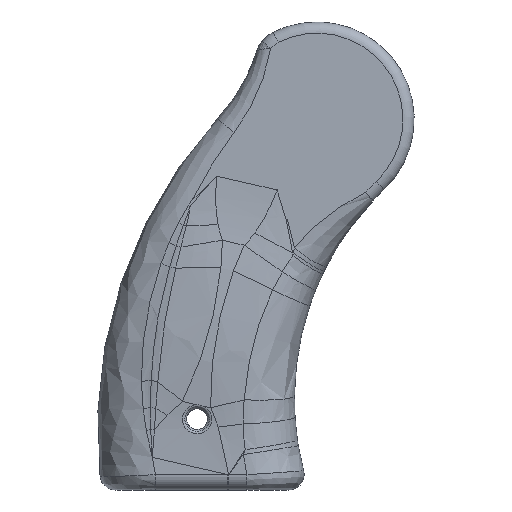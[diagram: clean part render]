
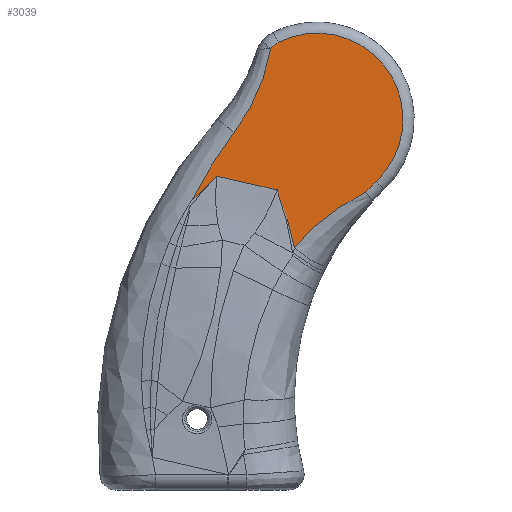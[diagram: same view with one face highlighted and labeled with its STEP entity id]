
A CAD part, front view. The second image highlights one B-rep face of the part: STEP entity #3039.
In plain terms, the highlighted planar face has unit normal (0, -1, 0).
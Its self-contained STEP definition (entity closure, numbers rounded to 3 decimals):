
#44=PLANE('',#3311);
#94=LINE('',#7707,#159);
#159=VECTOR('',#3801,10.);
#391=FACE_OUTER_BOUND('',#596,.T.);
#596=EDGE_LOOP('',(#2547,#2548,#2549,#2550,#2551,#2552,#2553,#2554,#2555,
#2556));
#791=B_SPLINE_CURVE_WITH_KNOTS('',3,(#7424,#7425,#7426,#7427,#7428,#7429),
 .UNSPECIFIED.,.F.,.F.,(4,2,4),(-1.76,-1.755,-0.68),
 .UNSPECIFIED.);
#835=B_SPLINE_CURVE_WITH_KNOTS('',3,(#8230,#8231,#8232,#8233,#8234),
 .UNSPECIFIED.,.F.,.F.,(4,1,4),(0.198,0.358,0.476),
 .UNSPECIFIED.);
#838=B_SPLINE_CURVE_WITH_KNOTS('',3,(#8290,#8291,#8292,#8293,#8294,#8295),
 .UNSPECIFIED.,.F.,.F.,(4,2,4),(-0.338,0.,1.319),
 .UNSPECIFIED.);
#848=B_SPLINE_CURVE_WITH_KNOTS('',3,(#8391,#8392,#8393,#8394),
 .UNSPECIFIED.,.F.,.F.,(4,4),(1.319,2.734),
 .UNSPECIFIED.);
#850=B_SPLINE_CURVE_WITH_KNOTS('',3,(#8456,#8457,#8458,#8459,#8460,#8461),
 .UNSPECIFIED.,.F.,.F.,(4,2,4),(0.142,0.227,0.228),
 .UNSPECIFIED.);
#851=B_SPLINE_CURVE_WITH_KNOTS('',3,(#8462,#8463,#8464,#8465,#8466,#8467),
 .UNSPECIFIED.,.F.,.F.,(4,2,4),(-0.507,0.,0.005),
 .UNSPECIFIED.);
#1024=CIRCLE('',#3304,15.352);
#1026=CIRCLE('',#3307,53.538);
#1028=CIRCLE('',#3310,4.);
#1262=VERTEX_POINT('',#7418);
#1263=VERTEX_POINT('',#7423);
#1282=VERTEX_POINT('',#7706);
#1298=VERTEX_POINT('',#8108);
#1299=VERTEX_POINT('',#8110);
#1300=VERTEX_POINT('',#8114);
#1301=VERTEX_POINT('',#8271);
#1302=VERTEX_POINT('',#8282);
#1311=VERTEX_POINT('',#8386);
#1312=VERTEX_POINT('',#8455);
#1665=EDGE_CURVE('',#1263,#1262,#791,.T.);
#1693=EDGE_CURVE('',#1282,#1263,#94,.T.);
#1721=EDGE_CURVE('',#1299,#1298,#1024,.T.);
#1724=EDGE_CURVE('',#1300,#1299,#1026,.T.);
#1725=EDGE_CURVE('',#1262,#1300,#835,.T.);
#1728=EDGE_CURVE('',#1301,#1302,#838,.T.);
#1738=EDGE_CURVE('',#1302,#1311,#848,.T.);
#1741=EDGE_CURVE('',#1298,#1301,#1028,.T.);
#1742=EDGE_CURVE('',#1312,#1311,#850,.T.);
#1743=EDGE_CURVE('',#1312,#1282,#851,.T.);
#2547=ORIENTED_EDGE('',*,*,#1742,.F.);
#2548=ORIENTED_EDGE('',*,*,#1743,.T.);
#2549=ORIENTED_EDGE('',*,*,#1693,.T.);
#2550=ORIENTED_EDGE('',*,*,#1665,.T.);
#2551=ORIENTED_EDGE('',*,*,#1725,.T.);
#2552=ORIENTED_EDGE('',*,*,#1724,.T.);
#2553=ORIENTED_EDGE('',*,*,#1721,.T.);
#2554=ORIENTED_EDGE('',*,*,#1741,.T.);
#2555=ORIENTED_EDGE('',*,*,#1728,.T.);
#2556=ORIENTED_EDGE('',*,*,#1738,.T.);
#3039=ADVANCED_FACE('',(#391),#44,.F.);
#3304=AXIS2_PLACEMENT_3D('',#8111,#3814,#3815);
#3307=AXIS2_PLACEMENT_3D('',#8194,#3820,#3821);
#3310=AXIS2_PLACEMENT_3D('',#8453,#3826,#3827);
#3311=AXIS2_PLACEMENT_3D('',#8454,#3828,#3829);
#3801=DIRECTION('',(0.975,0.,-0.222));
#3814=DIRECTION('center_axis',(0.,-1.,0.));
#3815=DIRECTION('ref_axis',(0.78,0.,0.626));
#3820=DIRECTION('center_axis',(0.,1.,0.));
#3821=DIRECTION('ref_axis',(0.69,0.,-0.724));
#3826=DIRECTION('center_axis',(0.,-1.,0.));
#3827=DIRECTION('ref_axis',(-0.63,0.,0.777));
#3828=DIRECTION('center_axis',(0.,1.,0.));
#3829=DIRECTION('ref_axis',(1.,0.,0.));
#7418=CARTESIAN_POINT('',(17.65,-6.75,40.273));
#7423=CARTESIAN_POINT('',(14.585,-6.75,50.63));
#7424=CARTESIAN_POINT('Ctrl Pts',(14.585,-6.75,50.63));
#7425=CARTESIAN_POINT('Ctrl Pts',(14.591,-6.75,50.615));
#7426=CARTESIAN_POINT('Ctrl Pts',(14.597,-6.75,50.599));
#7427=CARTESIAN_POINT('Ctrl Pts',(15.928,-6.75,47.255));
#7428=CARTESIAN_POINT('Ctrl Pts',(16.977,-6.75,43.794));
#7429=CARTESIAN_POINT('Ctrl Pts',(17.65,-6.75,40.273));
#7706=CARTESIAN_POINT('',(3.772,-6.75,53.09));
#7707=CARTESIAN_POINT('',(55.495,-6.75,41.32));
#8108=CARTESIAN_POINT('',(14.769,-6.75,76.947));
#8110=CARTESIAN_POINT('',(32.265,-6.75,52.123));
#8111=CARTESIAN_POINT('Origin',(21.67,-6.75,63.234));
#8114=CARTESIAN_POINT('',(30.358,-6.75,50.211));
#8194=CARTESIAN_POINT('Origin',(69.213,-6.75,13.378));
#8230=CARTESIAN_POINT('Ctrl Pts',(17.65,-6.75,40.273));
#8231=CARTESIAN_POINT('Ctrl Pts',(19.673,-6.75,42.723));
#8232=CARTESIAN_POINT('Ctrl Pts',(23.702,-6.75,46.489));
#8233=CARTESIAN_POINT('Ctrl Pts',(28.354,-6.75,49.219));
#8234=CARTESIAN_POINT('Ctrl Pts',(30.358,-6.75,50.211));
#8271=CARTESIAN_POINT('',(13.442,-6.75,75.871));
#8282=CARTESIAN_POINT('',(6.906,-6.75,60.88));
#8290=CARTESIAN_POINT('Ctrl Pts',(13.442,-6.75,75.871));
#8291=CARTESIAN_POINT('Ctrl Pts',(13.25,-6.75,74.759));
#8292=CARTESIAN_POINT('Ctrl Pts',(13.003,-6.75,73.662));
#8293=CARTESIAN_POINT('Ctrl Pts',(11.537,-6.75,68.359));
#8294=CARTESIAN_POINT('Ctrl Pts',(9.549,-6.75,64.371));
#8295=CARTESIAN_POINT('Ctrl Pts',(6.906,-6.75,60.88));
#8386=CARTESIAN_POINT('',(-0.54,-6.75,48.943));
#8391=CARTESIAN_POINT('Ctrl Pts',(6.906,-6.75,60.88));
#8392=CARTESIAN_POINT('Ctrl Pts',(4.072,-6.75,57.136));
#8393=CARTESIAN_POINT('Ctrl Pts',(1.577,-6.75,53.135));
#8394=CARTESIAN_POINT('Ctrl Pts',(-0.537,-6.75,48.942));
#8453=CARTESIAN_POINT('Origin',(16.567,-6.75,73.374));
#8454=CARTESIAN_POINT('Origin',(51.519,-6.75,24.406));
#8455=CARTESIAN_POINT('',(0.145,-6.75,49.461));
#8456=CARTESIAN_POINT('Ctrl Pts',(0.145,-6.75,49.461));
#8457=CARTESIAN_POINT('Ctrl Pts',(-0.074,-6.75,49.279));
#8458=CARTESIAN_POINT('Ctrl Pts',(-0.302,-6.75,49.105));
#8459=CARTESIAN_POINT('Ctrl Pts',(-0.536,-6.75,48.946));
#8460=CARTESIAN_POINT('Ctrl Pts',(-0.538,-6.75,48.945));
#8461=CARTESIAN_POINT('Ctrl Pts',(-0.54,-6.75,48.943));
#8462=CARTESIAN_POINT('Ctrl Pts',(0.145,-6.75,49.461));
#8463=CARTESIAN_POINT('Ctrl Pts',(1.291,-6.75,50.711));
#8464=CARTESIAN_POINT('Ctrl Pts',(2.493,-6.75,51.911));
#8465=CARTESIAN_POINT('Ctrl Pts',(3.749,-6.75,53.068));
#8466=CARTESIAN_POINT('Ctrl Pts',(3.76,-6.75,53.079));
#8467=CARTESIAN_POINT('Ctrl Pts',(3.772,-6.75,53.09));
